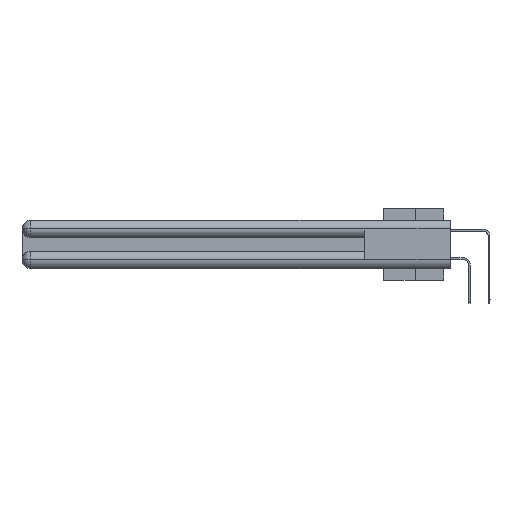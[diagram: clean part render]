
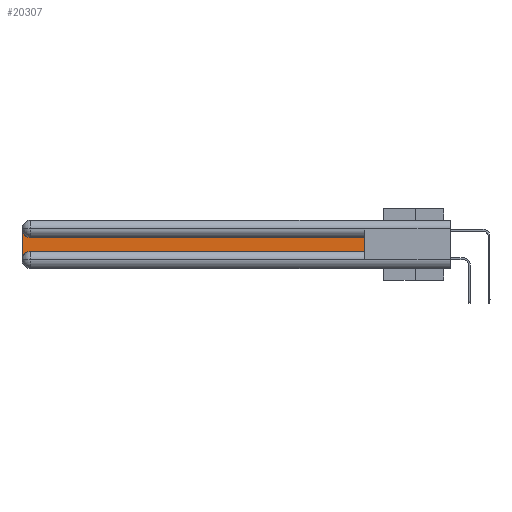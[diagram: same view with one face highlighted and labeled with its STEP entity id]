
A CAD part, left-side view. The second image highlights one B-rep face of the part: STEP entity #20307.
In plain terms, the highlighted planar face has unit normal (-1, 0, 0).
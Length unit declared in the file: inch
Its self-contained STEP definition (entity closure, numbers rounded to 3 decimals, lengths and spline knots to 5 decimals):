
#304 = EDGE_CURVE ( 'NONE', #38921, #33165, #14223, .T. ) ;
#497 = ORIENTED_EDGE ( 'NONE', *, *, #32205, .T. ) ;
#2889 = DIRECTION ( 'NONE',  ( 0., 0., -1. ) ) ;
#3957 = CARTESIAN_POINT ( 'NONE',  ( 0.075, 2.94, -0.0625 ) ) ;
#4757 = EDGE_CURVE ( 'NONE', #33165, #17172, #38446, .T. ) ;
#5744 = EDGE_CURVE ( 'NONE', #33836, #38921, #24313, .T. ) ;
#6051 = DIRECTION ( 'NONE',  ( 1., 0., 0. ) ) ;
#6936 = CARTESIAN_POINT ( 'NONE',  ( 0.075, 3., -0.1225 ) ) ;
#8798 = CARTESIAN_POINT ( 'NONE',  ( 0.075, 0.6, -0.1225 ) ) ;
#10047 = CARTESIAN_POINT ( 'NONE',  ( 0.075, 3., -0.2175 ) ) ;
#11286 = CARTESIAN_POINT ( 'NONE',  ( 0.075, 0.6, -0.2175 ) ) ;
#11548 = CARTESIAN_POINT ( 'NONE',  ( 0.075, 3., -0.2775 ) ) ;
#11562 = AXIS2_PLACEMENT_3D ( 'NONE', #6936, #15549, #38421 ) ;
#11748 = EDGE_LOOP ( 'NONE', ( #33233, #17874, #497, #34466, #23971, #19770 ) ) ;
#12332 = VECTOR ( 'NONE', #28982, 39.37008 ) ;
#14223 = LINE ( 'NONE', #11286, #18391 ) ;
#15255 = EDGE_CURVE ( 'NONE', #25351, #33836, #28732, .T. ) ;
#15549 = DIRECTION ( 'NONE',  ( 1., 0., 0. ) ) ;
#17172 = VERTEX_POINT ( 'NONE', #35759 ) ;
#17874 = ORIENTED_EDGE ( 'NONE', *, *, #27067, .T. ) ;
#18391 = VECTOR ( 'NONE', #30790, 39.37008 ) ;
#18899 = FACE_OUTER_BOUND ( 'NONE', #11748, .T. ) ;
#19700 = AXIS2_PLACEMENT_3D ( 'NONE', #3957, #38175, #29120 ) ;
#19770 = ORIENTED_EDGE ( 'NONE', *, *, #304, .T. ) ;
#20307 = ADVANCED_FACE ( 'NONE', ( #18899 ), #22674, .F. ) ;
#20436 = VECTOR ( 'NONE', #37109, 39.37008 ) ;
#21193 = CARTESIAN_POINT ( 'NONE',  ( 0.075, 3., -0.0625 ) ) ;
#22674 = PLANE ( 'NONE',  #11562 ) ;
#23971 = ORIENTED_EDGE ( 'NONE', *, *, #5744, .T. ) ;
#24313 = LINE ( 'NONE', #27865, #20436 ) ;
#24888 = CARTESIAN_POINT ( 'NONE',  ( 0.075, 2.94, -0.2175 ) ) ;
#25351 = VERTEX_POINT ( 'NONE', #11548 ) ;
#25534 = VERTEX_POINT ( 'NONE', #21193 ) ;
#25757 = CIRCLE ( 'NONE', #19700, 0.06 ) ;
#26369 = LINE ( 'NONE', #10047, #38037 ) ;
#26471 = CARTESIAN_POINT ( 'NONE',  ( 0.075, 0.6, -0.2175 ) ) ;
#26790 = DIRECTION ( 'NONE',  ( 0., 0., -1. ) ) ;
#27067 = EDGE_CURVE ( 'NONE', #17172, #25534, #25757, .T. ) ;
#27865 = CARTESIAN_POINT ( 'NONE',  ( 0.075, 0.6, -0.2175 ) ) ;
#28732 = CIRCLE ( 'NONE', #31430, 0.06 ) ;
#28982 = DIRECTION ( 'NONE',  ( 0., 1., 0. ) ) ;
#29120 = DIRECTION ( 'NONE',  ( 0., 0., -1. ) ) ;
#30790 = DIRECTION ( 'NONE',  ( 0., 0., 1. ) ) ;
#31430 = AXIS2_PLACEMENT_3D ( 'NONE', #34785, #6051, #2889 ) ;
#32205 = EDGE_CURVE ( 'NONE', #25534, #25351, #26369, .T. ) ;
#33165 = VERTEX_POINT ( 'NONE', #8798 ) ;
#33233 = ORIENTED_EDGE ( 'NONE', *, *, #4757, .T. ) ;
#33836 = VERTEX_POINT ( 'NONE', #24888 ) ;
#34466 = ORIENTED_EDGE ( 'NONE', *, *, #15255, .T. ) ;
#34785 = CARTESIAN_POINT ( 'NONE',  ( 0.075, 2.94, -0.2775 ) ) ;
#35759 = CARTESIAN_POINT ( 'NONE',  ( 0.075, 2.94, -0.1225 ) ) ;
#37109 = DIRECTION ( 'NONE',  ( 0., -1., 0. ) ) ;
#38037 = VECTOR ( 'NONE', #26790, 39.37008 ) ;
#38175 = DIRECTION ( 'NONE',  ( 1., 0., 0. ) ) ;
#38421 = DIRECTION ( 'NONE',  ( 0., 0., -1. ) ) ;
#38446 = LINE ( 'NONE', #38663, #12332 ) ;
#38663 = CARTESIAN_POINT ( 'NONE',  ( 0.075, 0.6, -0.1225 ) ) ;
#38921 = VERTEX_POINT ( 'NONE', #26471 ) ;
